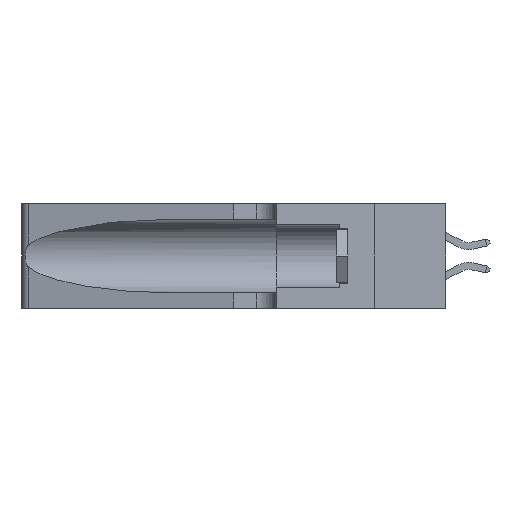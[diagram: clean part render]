
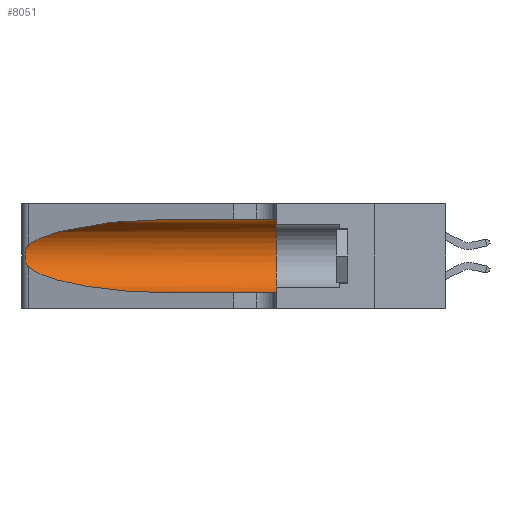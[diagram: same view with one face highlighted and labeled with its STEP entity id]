
A CAD part, left-side view. The second image highlights one B-rep face of the part: STEP entity #8051.
In plain terms, the highlighted cylindrical face has radius 3.308 mm (diameter 6.617 mm), a partial arc.
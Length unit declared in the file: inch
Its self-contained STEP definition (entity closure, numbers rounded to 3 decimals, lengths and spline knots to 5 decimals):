
#292 = ORIENTED_EDGE ( 'NONE', *, *, #14541, .T. ) ;
#930 = DIRECTION ( 'NONE',  ( 0., 0., -1. ) ) ;
#1114 = CARTESIAN_POINT ( 'NONE',  ( 0.25487, 1.22718, 0.14631 ) ) ;
#1526 = CARTESIAN_POINT ( 'NONE',  ( 0.26075, 1.23896, 0.178 ) ) ;
#1777 = CARTESIAN_POINT ( 'NONE',  ( 0.25854, 1.2359, 0.20912 ) ) ;
#3281 = CARTESIAN_POINT ( 'NONE',  ( 0.1305, 1.61858, 0.05475 ) ) ;
#3338 = DIRECTION ( 'NONE',  ( 0., -1., 0. ) ) ;
#3482 = CARTESIAN_POINT ( 'NONE',  ( 0.25555, 1.22994, 0.2215 ) ) ;
#3580 = CARTESIAN_POINT ( 'NONE',  ( 0.25487, 1.22718, 0.14631 ) ) ;
#4533 = CARTESIAN_POINT ( 'NONE',  ( 0.25487, 1.22718, 0.14631 ) ) ;
#4589 = VECTOR ( 'NONE', #10314, 39.37008 ) ;
#5240 = FACE_OUTER_BOUND ( 'NONE', #7453, .T. ) ;
#5504 = CARTESIAN_POINT ( 'NONE',  ( 0.25487, 1.22718, 0.22369 ) ) ;
#6137 = ORIENTED_EDGE ( 'NONE', *, *, #12328, .T. ) ;
#6374 = VERTEX_POINT ( 'NONE', #20602 ) ;
#6541 = CARTESIAN_POINT ( 'NONE',  ( 0.1305, 0.35, 0.31525 ) ) ;
#6864 = AXIS2_PLACEMENT_3D ( 'NONE', #25484, #18246, #18770 ) ;
#7031 = CARTESIAN_POINT ( 'NONE',  ( 0.1305, 0.35, 0.05475 ) ) ;
#7293 = EDGE_CURVE ( 'NONE', #22109, #25057, #18573, .T. ) ;
#7453 = EDGE_LOOP ( 'NONE', ( #292, #16851, #19595, #6137, #18323, #26142 ) ) ;
#7771 = CARTESIAN_POINT ( 'NONE',  ( 0.25787, 1.23484, 0.2124 ) ) ;
#8051 = ADVANCED_FACE ( 'NONE', ( #5240 ), #14414, .F. ) ;
#8197 = CARTESIAN_POINT ( 'NONE',  ( 0.1305, 1.61858, 0.31525 ) ) ;
#9585 = CARTESIAN_POINT ( 'NONE',  ( 0.2373, 1.15595, 0.28018 ) ) ;
#9631 = CARTESIAN_POINT ( 'NONE',  ( 0.25789, 1.23486, 0.15765 ) ) ;
#9711 = CARTESIAN_POINT ( 'NONE',  ( 0.25555, 1.22993, 0.14849 ) ) ;
#9795 = CARTESIAN_POINT ( 'NONE',  ( 0.26075, 1.23896, 0.19203 ) ) ;
#9878 = CARTESIAN_POINT ( 'NONE',  ( 0.25639, 1.23184, 0.21858 ) ) ;
#10314 = DIRECTION ( 'NONE',  ( 0., -1., 0. ) ) ;
#10877 = CARTESIAN_POINT ( 'NONE',  ( 0.1305, 1.61858, 0.185 ) ) ;
#11595 = CARTESIAN_POINT ( 'NONE',  ( 0.1305, 0.72297, 0.31525 ) ) ;
#12328 = EDGE_CURVE ( 'NONE', #6374, #25057, #22089, .T. ) ;
#12474 = AXIS2_PLACEMENT_3D ( 'NONE', #10877, #19021, #930 ) ;
#12525 = LINE ( 'NONE', #8197, #4589 ) ;
#12943 = EDGE_CURVE ( 'NONE', #21433, #22109, #12525, .T. ) ;
#13890 =( BOUNDED_CURVE ( )  B_SPLINE_CURVE ( 3, ( #11595, #21906, #9585, #5504 ),
 .UNSPECIFIED., .F., .T. ) 
 B_SPLINE_CURVE_WITH_KNOTS ( ( 4, 4 ),
 ( 1.5708, 2.84003 ),
 .UNSPECIFIED. ) 
 CURVE ( )  GEOMETRIC_REPRESENTATION_ITEM ( )  RATIONAL_B_SPLINE_CURVE ( ( 1., 0.87, 0.87, 1. ) ) 
 REPRESENTATION_ITEM ( '' )  );
#14265 = VERTEX_POINT ( 'NONE', #15488 ) ;
#14414 = CYLINDRICAL_SURFACE ( 'NONE', #12474, 0.13025 ) ;
#14541 = EDGE_CURVE ( 'NONE', #21433, #14265, #13890, .T. ) ;
#14853 = CARTESIAN_POINT ( 'NONE',  ( 0.1305, 0.72297, 0.31525 ) ) ;
#15488 = CARTESIAN_POINT ( 'NONE',  ( 0.25487, 1.22718, 0.22369 ) ) ;
#15851 =( BOUNDED_CURVE ( )  B_SPLINE_CURVE ( 3, ( #4533, #18530, #20674, #16653 ),
 .UNSPECIFIED., .F., .F. ) 
 B_SPLINE_CURVE_WITH_KNOTS ( ( 4, 4 ),
 ( 3.44316, 4.71239 ),
 .UNSPECIFIED. ) 
 CURVE ( )  GEOMETRIC_REPRESENTATION_ITEM ( )  RATIONAL_B_SPLINE_CURVE ( ( 1., 0.87, 0.87, 1. ) ) 
 REPRESENTATION_ITEM ( '' )  );
#16653 = CARTESIAN_POINT ( 'NONE',  ( 0.1305, 0.72297, 0.05475 ) ) ;
#16851 = ORIENTED_EDGE ( 'NONE', *, *, #18312, .T. ) ;
#18246 = DIRECTION ( 'NONE',  ( 0., 1., 0. ) ) ;
#18312 = EDGE_CURVE ( 'NONE', #14265, #24156, #21083, .T. ) ;
#18323 = ORIENTED_EDGE ( 'NONE', *, *, #7293, .F. ) ;
#18530 = CARTESIAN_POINT ( 'NONE',  ( 0.2373, 1.15595, 0.08982 ) ) ;
#18573 = CIRCLE ( 'NONE', #6864, 0.13025 ) ;
#18770 = DIRECTION ( 'NONE',  ( 0., 0., 1. ) ) ;
#19021 = DIRECTION ( 'NONE',  ( 0., -1., 0. ) ) ;
#19595 = ORIENTED_EDGE ( 'NONE', *, *, #23266, .T. ) ;
#19724 = CARTESIAN_POINT ( 'NONE',  ( 0.26017, 1.23833, 0.17102 ) ) ;
#19898 = CARTESIAN_POINT ( 'NONE',  ( 0.25856, 1.23593, 0.16098 ) ) ;
#20602 = CARTESIAN_POINT ( 'NONE',  ( 0.1305, 0.72297, 0.05475 ) ) ;
#20674 = CARTESIAN_POINT ( 'NONE',  ( 0.18966, 0.96281, 0.05475 ) ) ;
#21083 = B_SPLINE_CURVE_WITH_KNOTS ( 'NONE', 3,
 ( #21336, #3482, #9878, #7771, #1777, #24047, #9795, #1526, #19724, #19898, #9631, #21861, #9711, #3580 ),
 .UNSPECIFIED., .F., .F.,
 ( 4, 2, 2, 2, 2, 2, 4 ),
 ( 0., 0.00027, 0.00053, 0.00107, 0.0016, 0.00187, 0.00214 ),
 .UNSPECIFIED. ) ;
#21336 = CARTESIAN_POINT ( 'NONE',  ( 0.25487, 1.22718, 0.22369 ) ) ;
#21433 = VERTEX_POINT ( 'NONE', #14853 ) ;
#21861 = CARTESIAN_POINT ( 'NONE',  ( 0.25639, 1.23186, 0.15144 ) ) ;
#21906 = CARTESIAN_POINT ( 'NONE',  ( 0.18966, 0.96281, 0.31525 ) ) ;
#22089 = LINE ( 'NONE', #3281, #22705 ) ;
#22109 = VERTEX_POINT ( 'NONE', #6541 ) ;
#22705 = VECTOR ( 'NONE', #3338, 39.37008 ) ;
#23266 = EDGE_CURVE ( 'NONE', #24156, #6374, #15851, .T. ) ;
#24047 = CARTESIAN_POINT ( 'NONE',  ( 0.26018, 1.23835, 0.19895 ) ) ;
#24156 = VERTEX_POINT ( 'NONE', #1114 ) ;
#25057 = VERTEX_POINT ( 'NONE', #7031 ) ;
#25484 = CARTESIAN_POINT ( 'NONE',  ( 0.1305, 0.35, 0.185 ) ) ;
#26142 = ORIENTED_EDGE ( 'NONE', *, *, #12943, .F. ) ;
